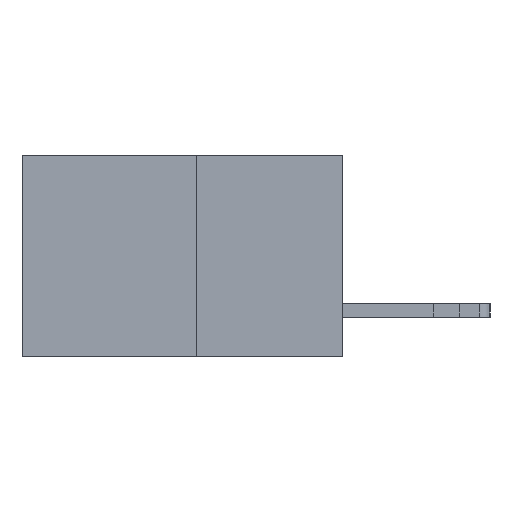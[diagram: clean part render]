
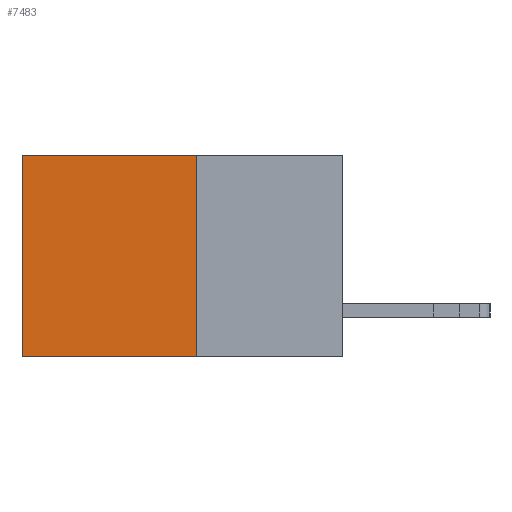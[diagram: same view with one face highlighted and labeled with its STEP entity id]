
A CAD part, left-side view. The second image highlights one B-rep face of the part: STEP entity #7483.
In plain terms, the highlighted planar face has unit normal (-1, 0, 0).
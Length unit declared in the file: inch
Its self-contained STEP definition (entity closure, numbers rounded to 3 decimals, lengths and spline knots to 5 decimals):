
#14 = CARTESIAN_POINT ( 'NONE',  ( 0.277, 0.27, -0.37 ) ) ;
#233 = CARTESIAN_POINT ( 'NONE',  ( 0.277, 0.27, -0.37 ) ) ;
#474 = EDGE_CURVE ( 'NONE', #28647, #1349, #18767, .T. ) ;
#1203 = DIRECTION ( 'NONE',  ( 1., 0., 0. ) ) ;
#1349 = VERTEX_POINT ( 'NONE', #5512 ) ;
#1388 = VERTEX_POINT ( 'NONE', #233 ) ;
#1614 = EDGE_CURVE ( 'NONE', #28647, #1388, #22346, .T. ) ;
#2824 = EDGE_CURVE ( 'NONE', #1349, #26371, #28507, .T. ) ;
#4377 = VECTOR ( 'NONE', #23462, 39.37008 ) ;
#5512 = CARTESIAN_POINT ( 'NONE',  ( 0.277, 0.59, 0. ) ) ;
#5629 = CARTESIAN_POINT ( 'NONE',  ( 0.277, 0.59, -0.37 ) ) ;
#7134 = EDGE_CURVE ( 'NONE', #1388, #26371, #25665, .T. ) ;
#7248 = CARTESIAN_POINT ( 'NONE',  ( 0.277, 0.27, 0. ) ) ;
#7483 = ADVANCED_FACE ( 'NONE', ( #26370 ), #17551, .F. ) ;
#7742 = VECTOR ( 'NONE', #22086, 39.37008 ) ;
#8201 = DIRECTION ( 'NONE',  ( 0., 0., -1. ) ) ;
#16570 = ORIENTED_EDGE ( 'NONE', *, *, #2824, .T. ) ;
#17517 = CARTESIAN_POINT ( 'NONE',  ( 0.277, 0.59, -0.37 ) ) ;
#17551 = PLANE ( 'NONE',  #28134 ) ;
#18004 = VECTOR ( 'NONE', #25617, 39.37008 ) ;
#18767 = LINE ( 'NONE', #26526, #7742 ) ;
#18769 = ORIENTED_EDGE ( 'NONE', *, *, #474, .T. ) ;
#19169 = EDGE_LOOP ( 'NONE', ( #16570, #20614, #25009, #18769 ) ) ;
#19889 = CARTESIAN_POINT ( 'NONE',  ( 0.277, 0.27, -0.37 ) ) ;
#20614 = ORIENTED_EDGE ( 'NONE', *, *, #7134, .F. ) ;
#21114 = DIRECTION ( 'NONE',  ( 0., 0., -1. ) ) ;
#21689 = CARTESIAN_POINT ( 'NONE',  ( 0.277, 0.27, -0.37 ) ) ;
#22086 = DIRECTION ( 'NONE',  ( 0., 1., 0. ) ) ;
#22262 = VECTOR ( 'NONE', #21114, 39.37008 ) ;
#22346 = LINE ( 'NONE', #21689, #4377 ) ;
#23462 = DIRECTION ( 'NONE',  ( 0., 0., -1. ) ) ;
#25009 = ORIENTED_EDGE ( 'NONE', *, *, #1614, .F. ) ;
#25617 = DIRECTION ( 'NONE',  ( 0., 1., 0. ) ) ;
#25665 = LINE ( 'NONE', #14, #18004 ) ;
#26370 = FACE_OUTER_BOUND ( 'NONE', #19169, .T. ) ;
#26371 = VERTEX_POINT ( 'NONE', #17517 ) ;
#26526 = CARTESIAN_POINT ( 'NONE',  ( 0.277, 0.27, 0. ) ) ;
#28134 = AXIS2_PLACEMENT_3D ( 'NONE', #19889, #1203, #8201 ) ;
#28507 = LINE ( 'NONE', #5629, #22262 ) ;
#28647 = VERTEX_POINT ( 'NONE', #7248 ) ;
